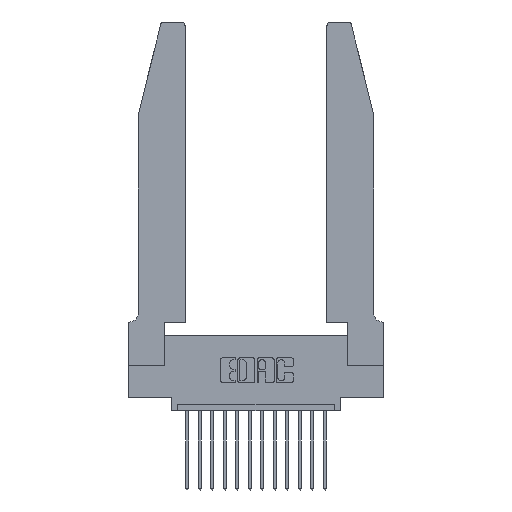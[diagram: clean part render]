
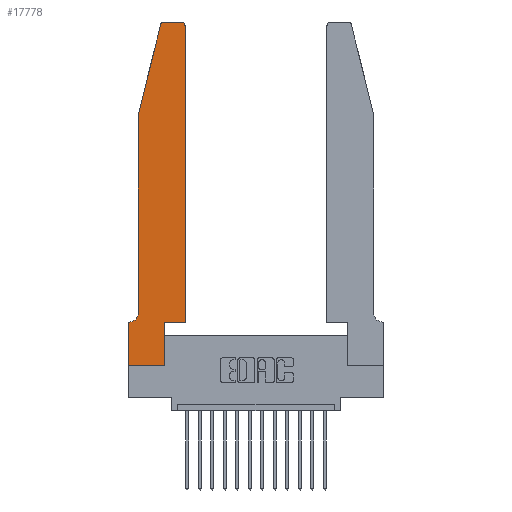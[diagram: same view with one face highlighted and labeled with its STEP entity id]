
A CAD part, top view. The second image highlights one B-rep face of the part: STEP entity #17778.
In plain terms, the highlighted planar face has unit normal (0, 0, 1).
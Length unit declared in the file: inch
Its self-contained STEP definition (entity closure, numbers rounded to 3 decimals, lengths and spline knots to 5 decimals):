
#94 = CARTESIAN_POINT ( 'NONE',  ( 0.4505, 0.35, 0.37 ) ) ;
#101 = DIRECTION ( 'NONE',  ( 1., 0., 0. ) ) ;
#208 = VECTOR ( 'NONE', #10557, 39.37008 ) ;
#290 = CARTESIAN_POINT ( 'NONE',  ( 0., 0., 0.37 ) ) ;
#492 = CIRCLE ( 'NONE', #4097, 0.07 ) ;
#556 = VERTEX_POINT ( 'NONE', #11810 ) ;
#611 = DIRECTION ( 'NONE',  ( 1., 0., 0. ) ) ;
#779 = LINE ( 'NONE', #15707, #17499 ) ;
#783 = CARTESIAN_POINT ( 'NONE',  ( 0.4505, 2.72, 0.37 ) ) ;
#821 = EDGE_CURVE ( 'NONE', #10088, #11328, #16490, .T. ) ;
#853 = DIRECTION ( 'NONE',  ( 0., -1., 0. ) ) ;
#1242 = VERTEX_POINT ( 'NONE', #13454 ) ;
#1365 = LINE ( 'NONE', #2768, #13058 ) ;
#1776 = EDGE_LOOP ( 'NONE', ( #2047, #4880, #17212, #6066, #7303, #15248, #10056, #16323, #7233, #17403, #12351, #10298 ) ) ;
#2040 = EDGE_CURVE ( 'NONE', #7394, #2971, #15771, .T. ) ;
#2047 = ORIENTED_EDGE ( 'NONE', *, *, #9640, .T. ) ;
#2185 = VERTEX_POINT ( 'NONE', #6756 ) ;
#2242 = CARTESIAN_POINT ( 'NONE',  ( 0., 0., 0.37 ) ) ;
#2532 = EDGE_CURVE ( 'NONE', #556, #3382, #16727, .T. ) ;
#2768 = CARTESIAN_POINT ( 'NONE',  ( 0.0755, 2., 0.37 ) ) ;
#2800 = CARTESIAN_POINT ( 'NONE',  ( 0.2865, 0.35, 0.37 ) ) ;
#2863 = VECTOR ( 'NONE', #17766, 39.37008 ) ;
#2971 = VERTEX_POINT ( 'NONE', #783 ) ;
#3140 = DIRECTION ( 'NONE',  ( 0., -1., 0. ) ) ;
#3169 = CARTESIAN_POINT ( 'NONE',  ( 0.0755, 2., 0.37 ) ) ;
#3382 = VERTEX_POINT ( 'NONE', #290 ) ;
#3400 = DIRECTION ( 'NONE',  ( 0., 0., 1. ) ) ;
#3521 = EDGE_CURVE ( 'NONE', #11328, #7394, #7402, .T. ) ;
#4097 = AXIS2_PLACEMENT_3D ( 'NONE', #13635, #6738, #15096 ) ;
#4858 = VECTOR ( 'NONE', #101, 39.37008 ) ;
#4880 = ORIENTED_EDGE ( 'NONE', *, *, #9195, .T. ) ;
#5533 = DIRECTION ( 'NONE',  ( 1., 0., 0. ) ) ;
#5861 = EDGE_CURVE ( 'NONE', #2971, #2185, #13182, .T. ) ;
#6066 = ORIENTED_EDGE ( 'NONE', *, *, #15529, .T. ) ;
#6132 = LINE ( 'NONE', #12403, #4858 ) ;
#6388 = CARTESIAN_POINT ( 'NONE',  ( 0.0055, 0.35, 0.37 ) ) ;
#6628 = VECTOR ( 'NONE', #11908, 39.37008 ) ;
#6738 = DIRECTION ( 'NONE',  ( 0., 0., -1. ) ) ;
#6756 = CARTESIAN_POINT ( 'NONE',  ( 0.4205, 2.75, 0.37 ) ) ;
#7233 = ORIENTED_EDGE ( 'NONE', *, *, #821, .T. ) ;
#7246 = DIRECTION ( 'NONE',  ( 0., 1., 0. ) ) ;
#7295 = CARTESIAN_POINT ( 'NONE',  ( 0.2605, 2.75, 0.37 ) ) ;
#7303 = ORIENTED_EDGE ( 'NONE', *, *, #15689, .T. ) ;
#7394 = VERTEX_POINT ( 'NONE', #94 ) ;
#7402 = LINE ( 'NONE', #14562, #6628 ) ;
#7422 = VERTEX_POINT ( 'NONE', #10800 ) ;
#7474 = DIRECTION ( 'NONE',  ( 1., 0., 0. ) ) ;
#7490 = CARTESIAN_POINT ( 'NONE',  ( 0.284, 2.75, 0.37 ) ) ;
#7643 = CARTESIAN_POINT ( 'NONE',  ( 0.4205, 2.72, 0.37 ) ) ;
#7669 = EDGE_CURVE ( 'NONE', #13022, #556, #779, .T. ) ;
#7906 = EDGE_CURVE ( 'NONE', #3382, #10088, #6132, .T. ) ;
#8822 = CARTESIAN_POINT ( 'NONE',  ( 0.2865, 0., 0.37 ) ) ;
#9195 = EDGE_CURVE ( 'NONE', #14121, #13513, #11543, .T. ) ;
#9416 = VECTOR ( 'NONE', #7246, 39.37008 ) ;
#9640 = EDGE_CURVE ( 'NONE', #2185, #14121, #17632, .T. ) ;
#9749 = VECTOR ( 'NONE', #853, 39.37008 ) ;
#9802 = AXIS2_PLACEMENT_3D ( 'NONE', #7643, #3400, #7474 ) ;
#10056 = ORIENTED_EDGE ( 'NONE', *, *, #2532, .T. ) ;
#10088 = VERTEX_POINT ( 'NONE', #8822 ) ;
#10104 = DIRECTION ( 'NONE',  ( 0., 0., 1. ) ) ;
#10298 = ORIENTED_EDGE ( 'NONE', *, *, #5861, .T. ) ;
#10557 = DIRECTION ( 'NONE',  ( 0., 1., 0. ) ) ;
#10800 = CARTESIAN_POINT ( 'NONE',  ( 0.0755, 0.42, 0.37 ) ) ;
#11328 = VERTEX_POINT ( 'NONE', #2800 ) ;
#11543 = CIRCLE ( 'NONE', #12895, 0.03 ) ;
#11589 = VECTOR ( 'NONE', #12852, 39.37008 ) ;
#11810 = CARTESIAN_POINT ( 'NONE',  ( 0., 0.35, 0.37 ) ) ;
#11908 = DIRECTION ( 'NONE',  ( 1., 0., 0. ) ) ;
#12351 = ORIENTED_EDGE ( 'NONE', *, *, #2040, .T. ) ;
#12403 = CARTESIAN_POINT ( 'NONE',  ( 0., 0., 0.37 ) ) ;
#12598 = CARTESIAN_POINT ( 'NONE',  ( 0.284, 2.72, 0.37 ) ) ;
#12793 = DIRECTION ( 'NONE',  ( -1., 0., 0. ) ) ;
#12852 = DIRECTION ( 'NONE',  ( -0.239, -0.971, 0. ) ) ;
#12895 = AXIS2_PLACEMENT_3D ( 'NONE', #12598, #16579, #5533 ) ;
#13022 = VERTEX_POINT ( 'NONE', #6388 ) ;
#13058 = VECTOR ( 'NONE', #3140, 39.37008 ) ;
#13182 = CIRCLE ( 'NONE', #9802, 0.03 ) ;
#13190 = FACE_OUTER_BOUND ( 'NONE', #1776, .T. ) ;
#13454 = CARTESIAN_POINT ( 'NONE',  ( 0.0755, 2., 0.37 ) ) ;
#13513 = VERTEX_POINT ( 'NONE', #15952 ) ;
#13635 = CARTESIAN_POINT ( 'NONE',  ( 0.0055, 0.42, 0.37 ) ) ;
#14121 = VERTEX_POINT ( 'NONE', #7490 ) ;
#14167 = LINE ( 'NONE', #3169, #11589 ) ;
#14348 = PLANE ( 'NONE',  #15400 ) ;
#14527 = EDGE_CURVE ( 'NONE', #13513, #1242, #14167, .T. ) ;
#14562 = CARTESIAN_POINT ( 'NONE',  ( 0.4505, 0.35, 0.37 ) ) ;
#15096 = DIRECTION ( 'NONE',  ( -1., 0., 0. ) ) ;
#15248 = ORIENTED_EDGE ( 'NONE', *, *, #7669, .T. ) ;
#15327 = CARTESIAN_POINT ( 'NONE',  ( 0.4505, 0.35, 0.37 ) ) ;
#15400 = AXIS2_PLACEMENT_3D ( 'NONE', #15765, #10104, #611 ) ;
#15529 = EDGE_CURVE ( 'NONE', #1242, #7422, #1365, .T. ) ;
#15689 = EDGE_CURVE ( 'NONE', #7422, #13022, #492, .T. ) ;
#15707 = CARTESIAN_POINT ( 'NONE',  ( 0.0755, 0.35, 0.37 ) ) ;
#15765 = CARTESIAN_POINT ( 'NONE',  ( 0., 0.35, 0.37 ) ) ;
#15771 = LINE ( 'NONE', #15327, #9416 ) ;
#15952 = CARTESIAN_POINT ( 'NONE',  ( 0.25487, 2.72718, 0.37 ) ) ;
#15978 = CARTESIAN_POINT ( 'NONE',  ( 0.2865, 0.35, 0.37 ) ) ;
#16323 = ORIENTED_EDGE ( 'NONE', *, *, #7906, .T. ) ;
#16490 = LINE ( 'NONE', #15978, #208 ) ;
#16579 = DIRECTION ( 'NONE',  ( 0., 0., 1. ) ) ;
#16727 = LINE ( 'NONE', #2242, #9749 ) ;
#17212 = ORIENTED_EDGE ( 'NONE', *, *, #14527, .T. ) ;
#17403 = ORIENTED_EDGE ( 'NONE', *, *, #3521, .T. ) ;
#17499 = VECTOR ( 'NONE', #12793, 39.37008 ) ;
#17632 = LINE ( 'NONE', #7295, #2863 ) ;
#17766 = DIRECTION ( 'NONE',  ( -1., 0., 0. ) ) ;
#17778 = ADVANCED_FACE ( 'NONE', ( #13190 ), #14348, .T. ) ;
